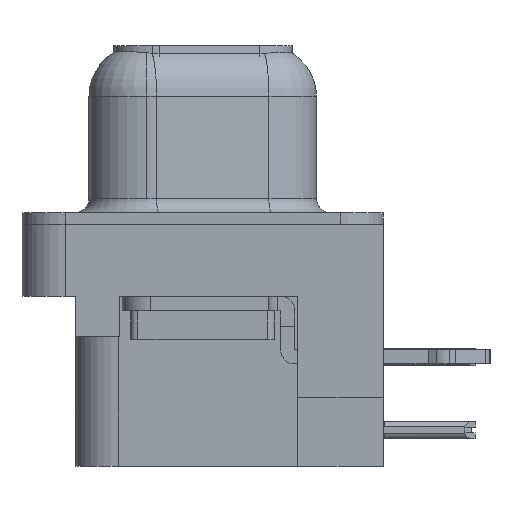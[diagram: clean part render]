
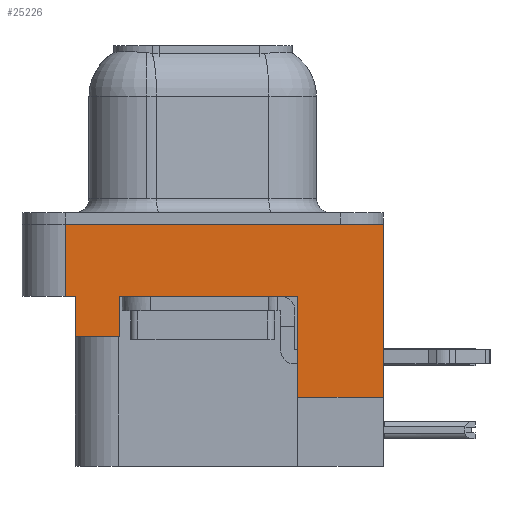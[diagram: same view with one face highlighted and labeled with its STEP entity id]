
A CAD part, left-side view. The second image highlights one B-rep face of the part: STEP entity #25226.
In plain terms, the highlighted planar face has unit normal (-1, 0, 0).
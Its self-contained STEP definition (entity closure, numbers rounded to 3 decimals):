
#116 = LINE ( 'NONE', #23508, #21202 ) ;
#542 = CARTESIAN_POINT ( 'NONE',  ( -2.935, 4.775, -2.5 ) ) ;
#849 = PLANE ( 'NONE',  #16600 ) ;
#1109 = DIRECTION ( 'NONE',  ( 0., -1., 0. ) ) ;
#1411 = VERTEX_POINT ( 'NONE', #14768 ) ;
#1549 = VECTOR ( 'NONE', #18412, 1000. ) ;
#1722 = CARTESIAN_POINT ( 'NONE',  ( -2.935, 4.425, -3.9 ) ) ;
#1994 = DIRECTION ( 'NONE',  ( 0., 0., 1. ) ) ;
#2275 = ORIENTED_EDGE ( 'NONE', *, *, #24148, .F. ) ;
#2320 = ORIENTED_EDGE ( 'NONE', *, *, #16984, .T. ) ;
#2907 = LINE ( 'NONE', #4510, #17908 ) ;
#3176 = CARTESIAN_POINT ( 'NONE',  ( -2.935, -6.275, -2.5 ) ) ;
#3361 = CARTESIAN_POINT ( 'NONE',  ( -2.935, 4.425, -2.5 ) ) ;
#3992 = VECTOR ( 'NONE', #16897, 1000. ) ;
#4089 = VECTOR ( 'NONE', #13957, 1000. ) ;
#4133 = CARTESIAN_POINT ( 'NONE',  ( -2.935, 4.425, -3.9 ) ) ;
#4510 = CARTESIAN_POINT ( 'NONE',  ( -2.935, -6.495, -6. ) ) ;
#4983 = DIRECTION ( 'NONE',  ( 0., 0., 1. ) ) ;
#5021 = ORIENTED_EDGE ( 'NONE', *, *, #21067, .F. ) ;
#5232 = LINE ( 'NONE', #15640, #16087 ) ;
#5384 = CARTESIAN_POINT ( 'NONE',  ( -2.935, 2.895, -3.9 ) ) ;
#5821 = ORIENTED_EDGE ( 'NONE', *, *, #21566, .T. ) ;
#6183 = CARTESIAN_POINT ( 'NONE',  ( -2.935, -6.275, -2.5 ) ) ;
#6559 = DIRECTION ( 'NONE',  ( 0., -1., 0. ) ) ;
#6643 = CARTESIAN_POINT ( 'NONE',  ( -2.935, -6.275, 0. ) ) ;
#6660 = VERTEX_POINT ( 'NONE', #14436 ) ;
#6671 = EDGE_LOOP ( 'NONE', ( #5021, #21672, #2275, #14710, #5821, #15513, #21364, #7224, #2320, #20710 ) ) ;
#7224 = ORIENTED_EDGE ( 'NONE', *, *, #18679, .T. ) ;
#7529 = FACE_OUTER_BOUND ( 'NONE', #6671, .T. ) ;
#8506 = VECTOR ( 'NONE', #6559, 1000. ) ;
#9393 = LINE ( 'NONE', #542, #3992 ) ;
#9501 = LINE ( 'NONE', #1722, #4089 ) ;
#10259 = VERTEX_POINT ( 'NONE', #12673 ) ;
#10337 = CARTESIAN_POINT ( 'NONE',  ( -2.935, -6.275, 0. ) ) ;
#12182 = CARTESIAN_POINT ( 'NONE',  ( -2.935, -3.295, -2.5 ) ) ;
#12189 = LINE ( 'NONE', #16300, #17646 ) ;
#12673 = CARTESIAN_POINT ( 'NONE',  ( -2.935, -6.275, -6. ) ) ;
#12690 = EDGE_CURVE ( 'NONE', #10259, #13540, #116, .T. ) ;
#12962 = CARTESIAN_POINT ( 'NONE',  ( -2.935, -3.295, -6. ) ) ;
#13540 = VERTEX_POINT ( 'NONE', #10337 ) ;
#13951 = LINE ( 'NONE', #6643, #8506 ) ;
#13957 = DIRECTION ( 'NONE',  ( 0., 1., 0. ) ) ;
#14354 = CARTESIAN_POINT ( 'NONE',  ( -2.935, 4.775, -2.5 ) ) ;
#14436 = CARTESIAN_POINT ( 'NONE',  ( -2.935, 4.775, 0. ) ) ;
#14710 = ORIENTED_EDGE ( 'NONE', *, *, #25652, .F. ) ;
#14768 = CARTESIAN_POINT ( 'NONE',  ( -2.935, 4.425, -3.9 ) ) ;
#15153 = CARTESIAN_POINT ( 'NONE',  ( -2.935, -6.275, -2.5 ) ) ;
#15513 = ORIENTED_EDGE ( 'NONE', *, *, #23431, .F. ) ;
#15547 = DIRECTION ( 'NONE',  ( 0., 0., 1. ) ) ;
#15640 = CARTESIAN_POINT ( 'NONE',  ( -2.935, -3.295, -8.4 ) ) ;
#15916 = VERTEX_POINT ( 'NONE', #24009 ) ;
#16087 = VECTOR ( 'NONE', #15547, 1000. ) ;
#16300 = CARTESIAN_POINT ( 'NONE',  ( -2.935, 2.895, -3.9 ) ) ;
#16536 = VECTOR ( 'NONE', #24527, 1000. ) ;
#16600 = AXIS2_PLACEMENT_3D ( 'NONE', #15153, #17206, #4983 ) ;
#16706 = DIRECTION ( 'NONE',  ( 0., 1., 0. ) ) ;
#16897 = DIRECTION ( 'NONE',  ( 0., 0., 1. ) ) ;
#16984 = EDGE_CURVE ( 'NONE', #15916, #19542, #17834, .T. ) ;
#17206 = DIRECTION ( 'NONE',  ( -1., 0., 0. ) ) ;
#17646 = VECTOR ( 'NONE', #1994, 1000. ) ;
#17834 = LINE ( 'NONE', #6183, #1549 ) ;
#17908 = VECTOR ( 'NONE', #16706, 1000. ) ;
#18412 = DIRECTION ( 'NONE',  ( 0., -1., 0. ) ) ;
#18534 = VERTEX_POINT ( 'NONE', #3361 ) ;
#18679 = EDGE_CURVE ( 'NONE', #23718, #15916, #12189, .T. ) ;
#19325 = EDGE_CURVE ( 'NONE', #20626, #19542, #5232, .T. ) ;
#19496 = DIRECTION ( 'NONE',  ( 0., 0., 1. ) ) ;
#19542 = VERTEX_POINT ( 'NONE', #12182 ) ;
#19791 = LINE ( 'NONE', #3176, #23294 ) ;
#20410 = VERTEX_POINT ( 'NONE', #14354 ) ;
#20626 = VERTEX_POINT ( 'NONE', #12962 ) ;
#20710 = ORIENTED_EDGE ( 'NONE', *, *, #19325, .F. ) ;
#21067 = EDGE_CURVE ( 'NONE', #10259, #20626, #2907, .T. ) ;
#21202 = VECTOR ( 'NONE', #19496, 1000. ) ;
#21364 = ORIENTED_EDGE ( 'NONE', *, *, #23285, .F. ) ;
#21566 = EDGE_CURVE ( 'NONE', #20410, #18534, #19791, .T. ) ;
#21672 = ORIENTED_EDGE ( 'NONE', *, *, #12690, .T. ) ;
#21928 = LINE ( 'NONE', #4133, #16536 ) ;
#23285 = EDGE_CURVE ( 'NONE', #23718, #1411, #9501, .T. ) ;
#23294 = VECTOR ( 'NONE', #1109, 1000. ) ;
#23431 = EDGE_CURVE ( 'NONE', #1411, #18534, #21928, .T. ) ;
#23508 = CARTESIAN_POINT ( 'NONE',  ( -2.935, -6.275, -2.5 ) ) ;
#23718 = VERTEX_POINT ( 'NONE', #5384 ) ;
#24009 = CARTESIAN_POINT ( 'NONE',  ( -2.935, 2.895, -2.5 ) ) ;
#24148 = EDGE_CURVE ( 'NONE', #6660, #13540, #13951, .T. ) ;
#24527 = DIRECTION ( 'NONE',  ( 0., 0., 1. ) ) ;
#25226 = ADVANCED_FACE ( 'NONE', ( #7529 ), #849, .T. ) ;
#25652 = EDGE_CURVE ( 'NONE', #20410, #6660, #9393, .T. ) ;
